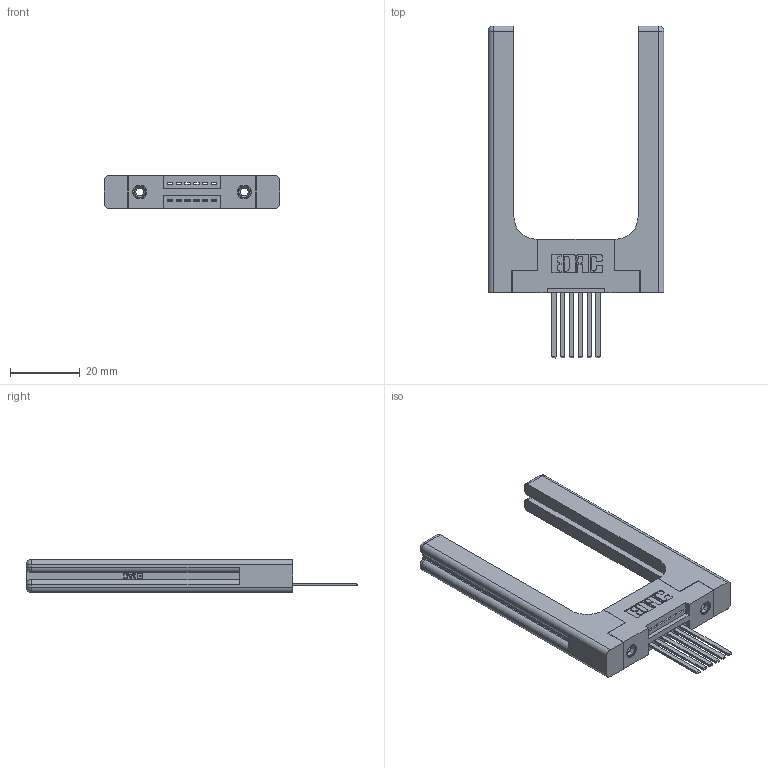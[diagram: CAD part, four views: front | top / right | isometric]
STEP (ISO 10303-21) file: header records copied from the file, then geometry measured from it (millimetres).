
FILE_DESCRIPTION (( 'STEP AP203' ), '1' );
FILE_NAME ('345-006-544-158.STEP', '2019-10-03T16:12:51', ( '' ), ( '' ), 'SwSTEP 2.0', 'SolidWorks 2016', '' );
FILE_SCHEMA (( 'CONFIG_CONTROL_DESIGN' ));
Length unit declared in the file: inch
Products named in the file (5): 345-006-544-158; 345 Part_Flush Mounting Lugs - 0.156 Dia-TH; 345-220-058_345-220-058; 345-292-001_345-293-144; 345-250-001_345-250-001-102
Assembly tree (11 placements, depth 2):
  345-006-544-158
    345 Part_Flush Mounting Lugs - 0.156 Dia-TH
    345-292-001_345-293-144  x6
    345-250-001_345-250-001-102  x2
    345-220-058_345-220-058  x2
Bounding box: 50.27 x 94.92 x 9.4 mm (x, y, z)
Volume: 13053.9 mm3; surface area: 11070.1 mm2
Topology: 11 solids, 11 shells, 694 faces, 1955 edges, 1274 vertices
Faces by surface type: plane 444, cylinder 190, bspline 36, cone 12, sphere 8, torus 4
Entity records: 14360 total; most frequent: CARTESIAN_POINT 3459, ORIENTED_EDGE 2196, DIRECTION 2018, EDGE_CURVE 1098, VECTOR 854, LINE 854, VERTEX_POINT 722, AXIS2_PLACEMENT_3D 582
